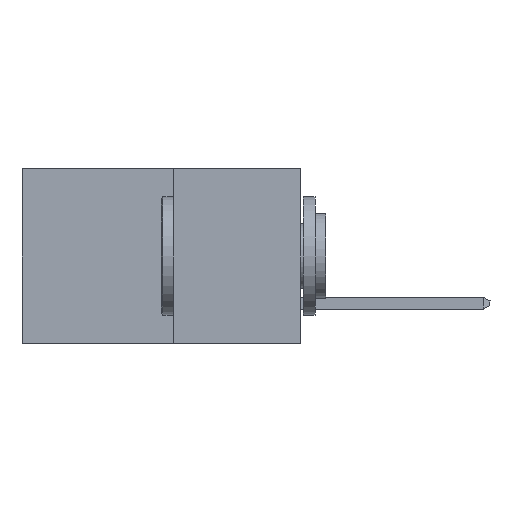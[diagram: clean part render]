
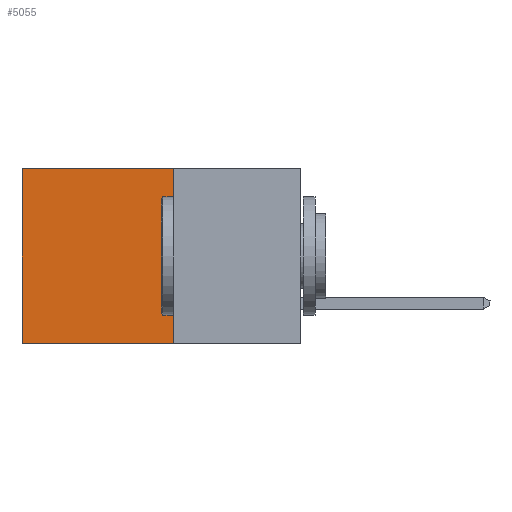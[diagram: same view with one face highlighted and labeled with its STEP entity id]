
A CAD part, left-side view. The second image highlights one B-rep face of the part: STEP entity #5055.
In plain terms, the highlighted planar face has unit normal (-1, 0, 0).
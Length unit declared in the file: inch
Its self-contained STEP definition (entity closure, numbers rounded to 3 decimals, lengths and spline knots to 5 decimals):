
#280 = LINE ( 'NONE', #7548, #2681 ) ;
#343 = EDGE_CURVE ( 'NONE', #7218, #11448, #6026, .T. ) ;
#616 = DIRECTION ( 'NONE',  ( 0., 1., 0. ) ) ;
#809 = EDGE_CURVE ( 'NONE', #7218, #10607, #6436, .T. ) ;
#1816 = EDGE_CURVE ( 'NONE', #11448, #8353, #9458, .T. ) ;
#1884 = VECTOR ( 'NONE', #10635, 39.37008 ) ;
#2681 = VECTOR ( 'NONE', #4746, 39.37008 ) ;
#3362 = ORIENTED_EDGE ( 'NONE', *, *, #343, .T. ) ;
#4746 = DIRECTION ( 'NONE',  ( 0., 1., 0. ) ) ;
#4769 = DIRECTION ( 'NONE',  ( 0., 0., -1. ) ) ;
#4876 = DIRECTION ( 'NONE',  ( 1., 0., 0. ) ) ;
#5055 = ADVANCED_FACE ( 'NONE', ( #5420 ), #5594, .F. ) ;
#5098 = CARTESIAN_POINT ( 'NONE',  ( 0.277, 0.27, -0.37 ) ) ;
#5310 = ORIENTED_EDGE ( 'NONE', *, *, #1816, .T. ) ;
#5420 = FACE_OUTER_BOUND ( 'NONE', #8464, .T. ) ;
#5594 = PLANE ( 'NONE',  #8275 ) ;
#6026 = LINE ( 'NONE', #7277, #10057 ) ;
#6436 = LINE ( 'NONE', #6915, #11206 ) ;
#6734 = DIRECTION ( 'NONE',  ( 0., 0., -1. ) ) ;
#6915 = CARTESIAN_POINT ( 'NONE',  ( 0.277, 0.27, -0.37 ) ) ;
#7218 = VERTEX_POINT ( 'NONE', #11283 ) ;
#7277 = CARTESIAN_POINT ( 'NONE',  ( 0.277, 0.27, 0. ) ) ;
#7548 = CARTESIAN_POINT ( 'NONE',  ( 0.277, 0.27, -0.37 ) ) ;
#7705 = CARTESIAN_POINT ( 'NONE',  ( 0.277, 0.59, -0.37 ) ) ;
#8084 = ORIENTED_EDGE ( 'NONE', *, *, #809, .F. ) ;
#8275 = AXIS2_PLACEMENT_3D ( 'NONE', #5098, #4876, #4769 ) ;
#8353 = VERTEX_POINT ( 'NONE', #7705 ) ;
#8464 = EDGE_LOOP ( 'NONE', ( #5310, #10219, #8084, #3362 ) ) ;
#8840 = CARTESIAN_POINT ( 'NONE',  ( 0.277, 0.59, 0. ) ) ;
#9458 = LINE ( 'NONE', #9507, #1884 ) ;
#9507 = CARTESIAN_POINT ( 'NONE',  ( 0.277, 0.59, -0.37 ) ) ;
#10057 = VECTOR ( 'NONE', #616, 39.37008 ) ;
#10219 = ORIENTED_EDGE ( 'NONE', *, *, #11833, .F. ) ;
#10607 = VERTEX_POINT ( 'NONE', #11821 ) ;
#10635 = DIRECTION ( 'NONE',  ( 0., 0., -1. ) ) ;
#11206 = VECTOR ( 'NONE', #6734, 39.37008 ) ;
#11283 = CARTESIAN_POINT ( 'NONE',  ( 0.277, 0.27, 0. ) ) ;
#11448 = VERTEX_POINT ( 'NONE', #8840 ) ;
#11821 = CARTESIAN_POINT ( 'NONE',  ( 0.277, 0.27, -0.37 ) ) ;
#11833 = EDGE_CURVE ( 'NONE', #10607, #8353, #280, .T. ) ;
